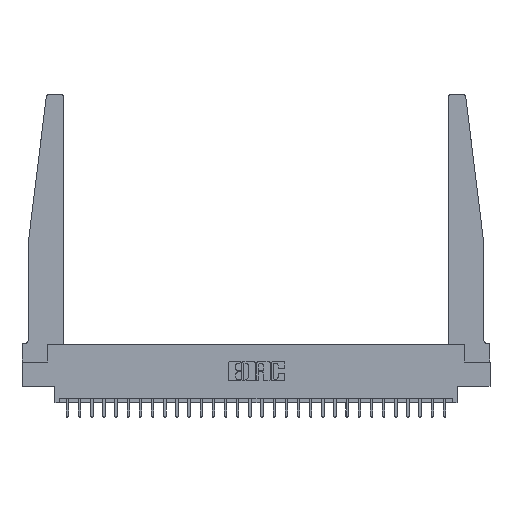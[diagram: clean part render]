
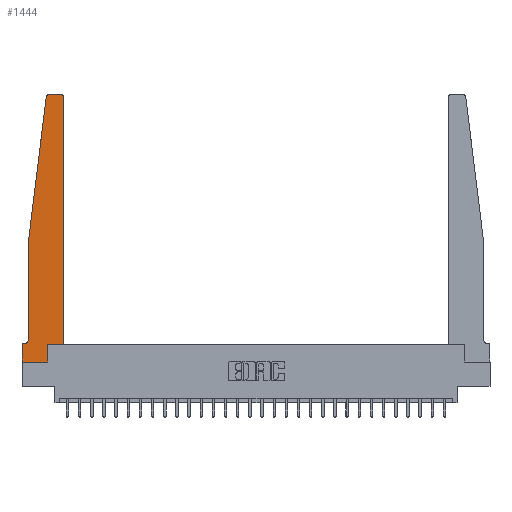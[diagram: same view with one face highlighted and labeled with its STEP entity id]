
A CAD part, top view. The second image highlights one B-rep face of the part: STEP entity #1444.
In plain terms, the highlighted planar face has unit normal (0, 0, 1).
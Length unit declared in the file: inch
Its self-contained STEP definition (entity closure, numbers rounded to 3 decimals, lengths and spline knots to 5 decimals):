
#123 = FACE_OUTER_BOUND ( 'NONE', #16568, .T. ) ;
#199 = VERTEX_POINT ( 'NONE', #14728 ) ;
#952 = EDGE_CURVE ( 'NONE', #17278, #5794, #17008, .T. ) ;
#1199 = CARTESIAN_POINT ( 'NONE',  ( 0.065, 1.25, 0.37 ) ) ;
#1283 = CARTESIAN_POINT ( 'NONE',  ( 0., 0., 0.37 ) ) ;
#1444 = ADVANCED_FACE ( 'NONE', ( #123 ), #18825, .T. ) ;
#3228 = VECTOR ( 'NONE', #6315, 39.37008 ) ;
#3650 = EDGE_CURVE ( 'NONE', #5794, #10838, #19469, .T. ) ;
#3675 = ORIENTED_EDGE ( 'NONE', *, *, #24714, .T. ) ;
#4066 = CARTESIAN_POINT ( 'NONE',  ( 0.2605, 0.18, 0.37 ) ) ;
#4296 = CARTESIAN_POINT ( 'NONE',  ( 0.015, 0.1875, 0.37 ) ) ;
#4315 = VECTOR ( 'NONE', #6201, 39.37008 ) ;
#4764 = VECTOR ( 'NONE', #16647, 39.37008 ) ;
#5048 = VECTOR ( 'NONE', #13808, 39.37008 ) ;
#5280 = CARTESIAN_POINT ( 'NONE',  ( 0., 0., 0.37 ) ) ;
#5342 = CARTESIAN_POINT ( 'NONE',  ( 0.065, 1.25, 0.37 ) ) ;
#5455 = VERTEX_POINT ( 'NONE', #22722 ) ;
#5794 = VERTEX_POINT ( 'NONE', #23191 ) ;
#5982 = VECTOR ( 'NONE', #19681, 39.37008 ) ;
#6201 = DIRECTION ( 'NONE',  ( 0., 1., 0. ) ) ;
#6315 = DIRECTION ( 'NONE',  ( 1., 0., 0. ) ) ;
#6458 = DIRECTION ( 'NONE',  ( 0., 0., 1. ) ) ;
#6756 = DIRECTION ( 'NONE',  ( 0., 0., -1. ) ) ;
#7176 = EDGE_CURVE ( 'NONE', #5455, #16090, #10306, .T. ) ;
#7405 = DIRECTION ( 'NONE',  ( 1., 0., 0. ) ) ;
#7667 = CIRCLE ( 'NONE', #7960, 0.03 ) ;
#7807 = CARTESIAN_POINT ( 'NONE',  ( 0.395, 2.75, 0.37 ) ) ;
#7960 = AXIS2_PLACEMENT_3D ( 'NONE', #18964, #6458, #21073 ) ;
#8237 = CARTESIAN_POINT ( 'NONE',  ( 0., 0.1875, 0.37 ) ) ;
#8351 = VERTEX_POINT ( 'NONE', #14605 ) ;
#8825 = DIRECTION ( 'NONE',  ( 0., 0., 1. ) ) ;
#9009 = ORIENTED_EDGE ( 'NONE', *, *, #13359, .T. ) ;
#9617 = DIRECTION ( 'NONE',  ( -0.122, -0.992, 0. ) ) ;
#9766 = CARTESIAN_POINT ( 'NONE',  ( 0.24675, 2.72367, 0.37 ) ) ;
#10182 = CARTESIAN_POINT ( 'NONE',  ( 0.425, 2.72, 0.37 ) ) ;
#10306 = LINE ( 'NONE', #10325, #4764 ) ;
#10325 = CARTESIAN_POINT ( 'NONE',  ( 0.425, 0.18, 0.37 ) ) ;
#10425 = CARTESIAN_POINT ( 'NONE',  ( 0., 0.1875, 0.37 ) ) ;
#10482 = EDGE_CURVE ( 'NONE', #16660, #5455, #19943, .T. ) ;
#10510 = DIRECTION ( 'NONE',  ( 1., 0., 0. ) ) ;
#10838 = VERTEX_POINT ( 'NONE', #9766 ) ;
#11001 = DIRECTION ( 'NONE',  ( -1., 0., 0. ) ) ;
#11213 = LINE ( 'NONE', #4066, #4315 ) ;
#11618 = LINE ( 'NONE', #1199, #17161 ) ;
#12220 = ORIENTED_EDGE ( 'NONE', *, *, #7176, .T. ) ;
#12712 = AXIS2_PLACEMENT_3D ( 'NONE', #21359, #8825, #23446 ) ;
#13359 = EDGE_CURVE ( 'NONE', #10838, #199, #14623, .T. ) ;
#13360 = VECTOR ( 'NONE', #7405, 39.37008 ) ;
#13650 = VERTEX_POINT ( 'NONE', #4296 ) ;
#13808 = DIRECTION ( 'NONE',  ( 0., -1., 0. ) ) ;
#14542 = ORIENTED_EDGE ( 'NONE', *, *, #25065, .T. ) ;
#14605 = CARTESIAN_POINT ( 'NONE',  ( 0.2605, 0., 0.37 ) ) ;
#14623 = LINE ( 'NONE', #5342, #19509 ) ;
#14728 = CARTESIAN_POINT ( 'NONE',  ( 0.065, 1.25, 0.37 ) ) ;
#15151 = CARTESIAN_POINT ( 'NONE',  ( 0.25, 2.75, 0.37 ) ) ;
#15598 = CARTESIAN_POINT ( 'NONE',  ( 0.065, 0.1875, 0.37 ) ) ;
#15959 = DIRECTION ( 'NONE',  ( 0., -1., 0. ) ) ;
#16090 = VERTEX_POINT ( 'NONE', #10182 ) ;
#16355 = VECTOR ( 'NONE', #11001, 39.37008 ) ;
#16451 = LINE ( 'NONE', #15598, #5982 ) ;
#16568 = EDGE_LOOP ( 'NONE', ( #22913, #26644, #9009, #21785, #26802, #19687, #3675, #21557, #27113, #20282, #12220, #14542 ) ) ;
#16647 = DIRECTION ( 'NONE',  ( 0., 1., 0. ) ) ;
#16660 = VERTEX_POINT ( 'NONE', #18284 ) ;
#16722 = CARTESIAN_POINT ( 'NONE',  ( 0.425, 0.18, 0.37 ) ) ;
#17008 = LINE ( 'NONE', #15151, #16355 ) ;
#17161 = VECTOR ( 'NONE', #15959, 39.37008 ) ;
#17278 = VERTEX_POINT ( 'NONE', #7807 ) ;
#17412 = VERTEX_POINT ( 'NONE', #8237 ) ;
#18284 = CARTESIAN_POINT ( 'NONE',  ( 0.2605, 0.18, 0.37 ) ) ;
#18458 = EDGE_CURVE ( 'NONE', #23548, #8351, #18892, .T. ) ;
#18782 = CIRCLE ( 'NONE', #25323, 0.05 ) ;
#18825 = PLANE ( 'NONE',  #23339 ) ;
#18892 = LINE ( 'NONE', #5280, #13360 ) ;
#18964 = CARTESIAN_POINT ( 'NONE',  ( 0.395, 2.72, 0.37 ) ) ;
#19253 = CARTESIAN_POINT ( 'NONE',  ( 0.015, 0.2375, 0.37 ) ) ;
#19469 = CIRCLE ( 'NONE', #12712, 0.03 ) ;
#19509 = VECTOR ( 'NONE', #9617, 39.37008 ) ;
#19681 = DIRECTION ( 'NONE',  ( -1., 0., 0. ) ) ;
#19687 = ORIENTED_EDGE ( 'NONE', *, *, #25369, .T. ) ;
#19943 = LINE ( 'NONE', #16722, #3228 ) ;
#20282 = ORIENTED_EDGE ( 'NONE', *, *, #10482, .T. ) ;
#20960 = VERTEX_POINT ( 'NONE', #24108 ) ;
#21055 = LINE ( 'NONE', #26229, #5048 ) ;
#21073 = DIRECTION ( 'NONE',  ( 1., 0., 0. ) ) ;
#21243 = EDGE_CURVE ( 'NONE', #20960, #13650, #18782, .T. ) ;
#21359 = CARTESIAN_POINT ( 'NONE',  ( 0.27653, 2.72, 0.37 ) ) ;
#21371 = DIRECTION ( 'NONE',  ( -1., 0., 0. ) ) ;
#21557 = ORIENTED_EDGE ( 'NONE', *, *, #18458, .T. ) ;
#21572 = EDGE_CURVE ( 'NONE', #199, #20960, #11618, .T. ) ;
#21785 = ORIENTED_EDGE ( 'NONE', *, *, #21572, .T. ) ;
#22722 = CARTESIAN_POINT ( 'NONE',  ( 0.425, 0.18, 0.37 ) ) ;
#22790 = EDGE_CURVE ( 'NONE', #8351, #16660, #11213, .T. ) ;
#22913 = ORIENTED_EDGE ( 'NONE', *, *, #952, .T. ) ;
#23041 = DIRECTION ( 'NONE',  ( 0., 0., 1. ) ) ;
#23191 = CARTESIAN_POINT ( 'NONE',  ( 0.27653, 2.75, 0.37 ) ) ;
#23339 = AXIS2_PLACEMENT_3D ( 'NONE', #10425, #23041, #10510 ) ;
#23446 = DIRECTION ( 'NONE',  ( 1., 0., 0. ) ) ;
#23548 = VERTEX_POINT ( 'NONE', #1283 ) ;
#24108 = CARTESIAN_POINT ( 'NONE',  ( 0.065, 0.2375, 0.37 ) ) ;
#24714 = EDGE_CURVE ( 'NONE', #17412, #23548, #21055, .T. ) ;
#25065 = EDGE_CURVE ( 'NONE', #16090, #17278, #7667, .T. ) ;
#25323 = AXIS2_PLACEMENT_3D ( 'NONE', #19253, #6756, #21371 ) ;
#25369 = EDGE_CURVE ( 'NONE', #13650, #17412, #16451, .T. ) ;
#26229 = CARTESIAN_POINT ( 'NONE',  ( 0., 0., 0.37 ) ) ;
#26644 = ORIENTED_EDGE ( 'NONE', *, *, #3650, .T. ) ;
#26802 = ORIENTED_EDGE ( 'NONE', *, *, #21243, .T. ) ;
#27113 = ORIENTED_EDGE ( 'NONE', *, *, #22790, .T. ) ;
